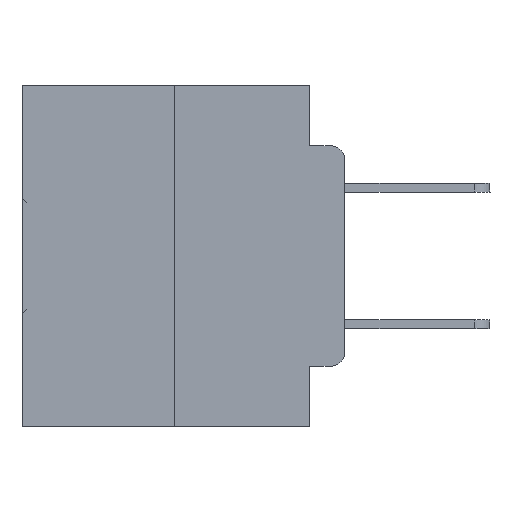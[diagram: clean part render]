
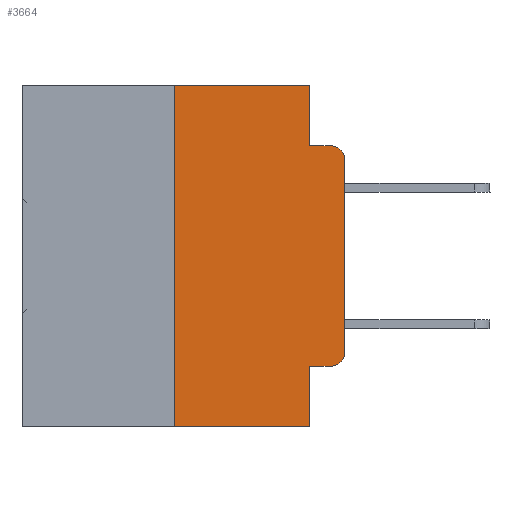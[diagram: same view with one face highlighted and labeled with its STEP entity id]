
A CAD part, left-side view. The second image highlights one B-rep face of the part: STEP entity #3664.
In plain terms, the highlighted planar face has unit normal (-1, 0, 0).
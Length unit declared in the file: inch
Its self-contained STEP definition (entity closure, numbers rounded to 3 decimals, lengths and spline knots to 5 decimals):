
#453 = CIRCLE ( 'NONE', #2494, 0.02 ) ;
#1198 = FACE_OUTER_BOUND ( 'NONE', #31324, .T. ) ;
#1498 = CIRCLE ( 'NONE', #15103, 0.02 ) ;
#1779 = VERTEX_POINT ( 'NONE', #20678 ) ;
#2206 = CARTESIAN_POINT ( 'NONE',  ( 0., 0.051, -0.4115 ) ) ;
#2494 = AXIS2_PLACEMENT_3D ( 'NONE', #4079, #22799, #14581 ) ;
#2608 = DIRECTION ( 'NONE',  ( 0., 0., -1. ) ) ;
#2957 = CARTESIAN_POINT ( 'NONE',  ( 0., 0.051, 0. ) ) ;
#2995 = CARTESIAN_POINT ( 'NONE',  ( 0., 0.473, -0.5 ) ) ;
#3232 = DIRECTION ( 'NONE',  ( 0., -1., 0. ) ) ;
#3664 = ADVANCED_FACE ( 'NONE', ( #1198 ), #33590, .F. ) ;
#3750 = DIRECTION ( 'NONE',  ( 0., 0., 1. ) ) ;
#3923 = ORIENTED_EDGE ( 'NONE', *, *, #5014, .T. ) ;
#4079 = CARTESIAN_POINT ( 'NONE',  ( 0., 0.02, -0.1085 ) ) ;
#4286 = ORIENTED_EDGE ( 'NONE', *, *, #6726, .F. ) ;
#4300 = ORIENTED_EDGE ( 'NONE', *, *, #10722, .F. ) ;
#4316 = LINE ( 'NONE', #32664, #24835 ) ;
#4647 = LINE ( 'NONE', #30133, #10902 ) ;
#5014 = EDGE_CURVE ( 'NONE', #5084, #1779, #1498, .T. ) ;
#5084 = VERTEX_POINT ( 'NONE', #15484 ) ;
#5736 = VERTEX_POINT ( 'NONE', #19550 ) ;
#5825 = VECTOR ( 'NONE', #3232, 39.37008 ) ;
#6301 = CARTESIAN_POINT ( 'NONE',  ( 0., 0.25, 0. ) ) ;
#6726 = EDGE_CURVE ( 'NONE', #9922, #12906, #4316, .T. ) ;
#7060 = DIRECTION ( 'NONE',  ( 0., 0., -1. ) ) ;
#7144 = CARTESIAN_POINT ( 'NONE',  ( 0., 0.051, -0.5 ) ) ;
#7350 = LINE ( 'NONE', #2206, #19117 ) ;
#7953 = LINE ( 'NONE', #8082, #32277 ) ;
#8082 = CARTESIAN_POINT ( 'NONE',  ( 0., 0., 0. ) ) ;
#8367 = EDGE_CURVE ( 'NONE', #5736, #13595, #4647, .T. ) ;
#9570 = CARTESIAN_POINT ( 'NONE',  ( 0., 0.473, 0. ) ) ;
#9893 = DIRECTION ( 'NONE',  ( 0., -1., 0. ) ) ;
#9922 = VERTEX_POINT ( 'NONE', #23355 ) ;
#10063 = DIRECTION ( 'NONE',  ( 0., 0., -1. ) ) ;
#10722 = EDGE_CURVE ( 'NONE', #13595, #9922, #28301, .T. ) ;
#10818 = ORIENTED_EDGE ( 'NONE', *, *, #8367, .F. ) ;
#10902 = VECTOR ( 'NONE', #21847, 39.37008 ) ;
#11016 = ORIENTED_EDGE ( 'NONE', *, *, #14389, .F. ) ;
#11361 = VERTEX_POINT ( 'NONE', #16945 ) ;
#12785 = CARTESIAN_POINT ( 'NONE',  ( 0., 0.051, 0. ) ) ;
#12894 = LINE ( 'NONE', #2995, #5825 ) ;
#12906 = VERTEX_POINT ( 'NONE', #14553 ) ;
#13283 = EDGE_CURVE ( 'NONE', #1779, #11361, #7953, .T. ) ;
#13595 = VERTEX_POINT ( 'NONE', #12785 ) ;
#13973 = VERTEX_POINT ( 'NONE', #25236 ) ;
#14136 = VERTEX_POINT ( 'NONE', #7144 ) ;
#14389 = EDGE_CURVE ( 'NONE', #13973, #14136, #28483, .T. ) ;
#14553 = CARTESIAN_POINT ( 'NONE',  ( 0., 0.02, -0.0885 ) ) ;
#14581 = DIRECTION ( 'NONE',  ( 0., 0., -1. ) ) ;
#15103 = AXIS2_PLACEMENT_3D ( 'NONE', #26524, #21256, #10063 ) ;
#15309 = EDGE_CURVE ( 'NONE', #11361, #12906, #453, .T. ) ;
#15484 = CARTESIAN_POINT ( 'NONE',  ( 0., 0.02, -0.4115 ) ) ;
#15708 = EDGE_CURVE ( 'NONE', #23315, #14136, #12894, .T. ) ;
#16185 = DIRECTION ( 'NONE',  ( 0., 0., 1. ) ) ;
#16358 = ORIENTED_EDGE ( 'NONE', *, *, #15708, .T. ) ;
#16504 = LINE ( 'NONE', #6301, #20277 ) ;
#16945 = CARTESIAN_POINT ( 'NONE',  ( 0., 0., -0.1085 ) ) ;
#17493 = CARTESIAN_POINT ( 'NONE',  ( 0., 0.051, 0. ) ) ;
#18224 = EDGE_CURVE ( 'NONE', #23315, #5736, #16504, .T. ) ;
#19117 = VECTOR ( 'NONE', #9893, 39.37008 ) ;
#19550 = CARTESIAN_POINT ( 'NONE',  ( 0., 0.25, 0. ) ) ;
#19638 = CARTESIAN_POINT ( 'NONE',  ( 0., 0.25, -0.5 ) ) ;
#20277 = VECTOR ( 'NONE', #3750, 39.37008 ) ;
#20678 = CARTESIAN_POINT ( 'NONE',  ( 0., 0., -0.3915 ) ) ;
#21256 = DIRECTION ( 'NONE',  ( -1., 0., 0. ) ) ;
#21847 = DIRECTION ( 'NONE',  ( 0., -1., 0. ) ) ;
#22349 = EDGE_CURVE ( 'NONE', #13973, #5084, #7350, .T. ) ;
#22799 = DIRECTION ( 'NONE',  ( -1., 0., 0. ) ) ;
#23315 = VERTEX_POINT ( 'NONE', #19638 ) ;
#23355 = CARTESIAN_POINT ( 'NONE',  ( 0., 0.051, -0.0885 ) ) ;
#24835 = VECTOR ( 'NONE', #32441, 39.37008 ) ;
#25236 = CARTESIAN_POINT ( 'NONE',  ( 0., 0.051, -0.4115 ) ) ;
#26192 = VECTOR ( 'NONE', #7060, 39.37008 ) ;
#26524 = CARTESIAN_POINT ( 'NONE',  ( 0., 0.02, -0.3915 ) ) ;
#26640 = ORIENTED_EDGE ( 'NONE', *, *, #18224, .F. ) ;
#27253 = VECTOR ( 'NONE', #2608, 39.37008 ) ;
#28301 = LINE ( 'NONE', #17493, #26192 ) ;
#28483 = LINE ( 'NONE', #2957, #27253 ) ;
#30133 = CARTESIAN_POINT ( 'NONE',  ( 0., 0.473, 0. ) ) ;
#31324 = EDGE_LOOP ( 'NONE', ( #33221, #34498, #4286, #4300, #10818, #26640, #16358, #11016, #32982, #3923 ) ) ;
#32277 = VECTOR ( 'NONE', #16185, 39.37008 ) ;
#32441 = DIRECTION ( 'NONE',  ( 0., -1., 0. ) ) ;
#32664 = CARTESIAN_POINT ( 'NONE',  ( 0., 0.051, -0.0885 ) ) ;
#32982 = ORIENTED_EDGE ( 'NONE', *, *, #22349, .T. ) ;
#33221 = ORIENTED_EDGE ( 'NONE', *, *, #13283, .T. ) ;
#33254 = DIRECTION ( 'NONE',  ( 0., 0., -1. ) ) ;
#33370 = DIRECTION ( 'NONE',  ( 1., 0., 0. ) ) ;
#33590 = PLANE ( 'NONE',  #33854 ) ;
#33854 = AXIS2_PLACEMENT_3D ( 'NONE', #9570, #33370, #33254 ) ;
#34498 = ORIENTED_EDGE ( 'NONE', *, *, #15309, .T. ) ;
